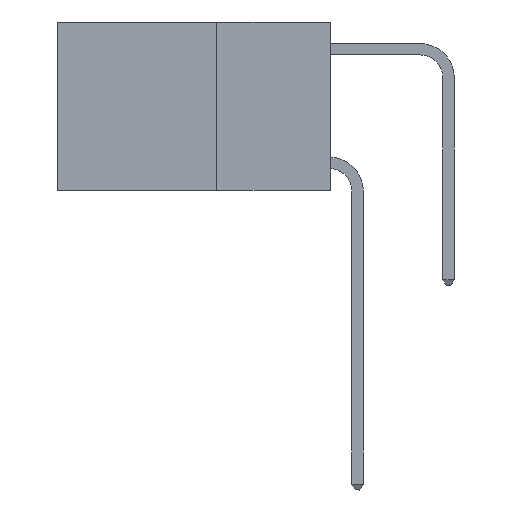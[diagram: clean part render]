
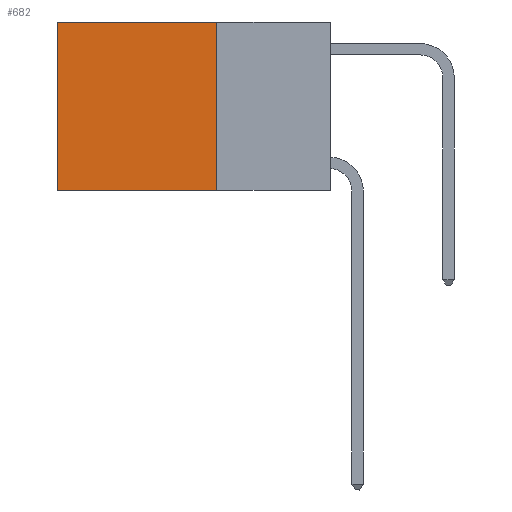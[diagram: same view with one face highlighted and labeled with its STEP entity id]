
A CAD part, left-side view. The second image highlights one B-rep face of the part: STEP entity #682.
In plain terms, the highlighted planar face has unit normal (-1, 0, 0).
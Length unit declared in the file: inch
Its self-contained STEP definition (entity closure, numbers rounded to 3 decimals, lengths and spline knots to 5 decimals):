
#162 = DIRECTION ( 'NONE',  ( 0., 0., -1. ) ) ;
#268 = FACE_OUTER_BOUND ( 'NONE', #15762, .T. ) ;
#305 = VERTEX_POINT ( 'NONE', #2105 ) ;
#682 = ADVANCED_FACE ( 'NONE', ( #268 ), #12542, .F. ) ;
#943 = AXIS2_PLACEMENT_3D ( 'NONE', #15079, #7830, #8630 ) ;
#982 = EDGE_CURVE ( 'NONE', #9145, #17324, #10990, .T. ) ;
#1053 = VECTOR ( 'NONE', #13660, 39.37008 ) ;
#2105 = CARTESIAN_POINT ( 'NONE',  ( 0.2625, 0.6, 0. ) ) ;
#3466 = DIRECTION ( 'NONE',  ( 0., 1., 0. ) ) ;
#4491 = VECTOR ( 'NONE', #8944, 39.37008 ) ;
#4861 = CARTESIAN_POINT ( 'NONE',  ( 0.2625, 0.6, 0. ) ) ;
#5264 = LINE ( 'NONE', #13591, #1053 ) ;
#6143 = VECTOR ( 'NONE', #162, 39.37008 ) ;
#6889 = VECTOR ( 'NONE', #3466, 39.37008 ) ;
#7830 = DIRECTION ( 'NONE',  ( 1., 0., 0. ) ) ;
#8265 = VERTEX_POINT ( 'NONE', #15396 ) ;
#8630 = DIRECTION ( 'NONE',  ( 0., 0., -1. ) ) ;
#8944 = DIRECTION ( 'NONE',  ( 0., 0., -1. ) ) ;
#9093 = LINE ( 'NONE', #18057, #4491 ) ;
#9145 = VERTEX_POINT ( 'NONE', #15881 ) ;
#10734 = LINE ( 'NONE', #4861, #6143 ) ;
#10990 = LINE ( 'NONE', #19864, #6889 ) ;
#11169 = ORIENTED_EDGE ( 'NONE', *, *, #982, .F. ) ;
#11769 = ORIENTED_EDGE ( 'NONE', *, *, #14869, .T. ) ;
#12072 = ORIENTED_EDGE ( 'NONE', *, *, #16423, .T. ) ;
#12542 = PLANE ( 'NONE',  #943 ) ;
#13591 = CARTESIAN_POINT ( 'NONE',  ( 0.2625, 0.25, 0. ) ) ;
#13660 = DIRECTION ( 'NONE',  ( 0., 1., 0. ) ) ;
#14869 = EDGE_CURVE ( 'NONE', #8265, #305, #5264, .T. ) ;
#15079 = CARTESIAN_POINT ( 'NONE',  ( 0.2625, 0.25, 0. ) ) ;
#15396 = CARTESIAN_POINT ( 'NONE',  ( 0.2625, 0.25, 0. ) ) ;
#15548 = EDGE_CURVE ( 'NONE', #8265, #9145, #9093, .T. ) ;
#15762 = EDGE_LOOP ( 'NONE', ( #12072, #11169, #16116, #11769 ) ) ;
#15881 = CARTESIAN_POINT ( 'NONE',  ( 0.2625, 0.25, -0.37 ) ) ;
#16116 = ORIENTED_EDGE ( 'NONE', *, *, #15548, .F. ) ;
#16423 = EDGE_CURVE ( 'NONE', #305, #17324, #10734, .T. ) ;
#17324 = VERTEX_POINT ( 'NONE', #17980 ) ;
#17980 = CARTESIAN_POINT ( 'NONE',  ( 0.2625, 0.6, -0.37 ) ) ;
#18057 = CARTESIAN_POINT ( 'NONE',  ( 0.2625, 0.25, 0. ) ) ;
#19864 = CARTESIAN_POINT ( 'NONE',  ( 0.2625, 0.25, -0.37 ) ) ;
